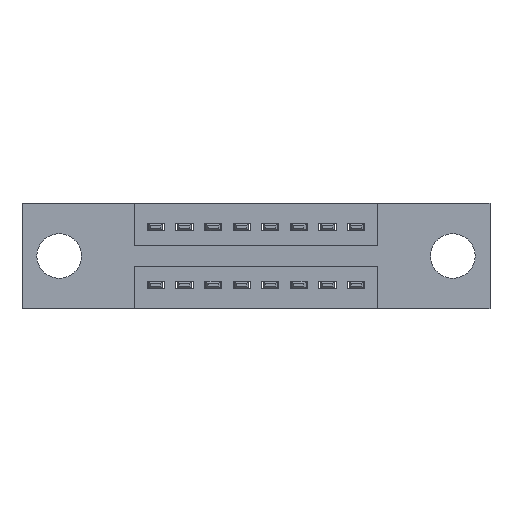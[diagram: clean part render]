
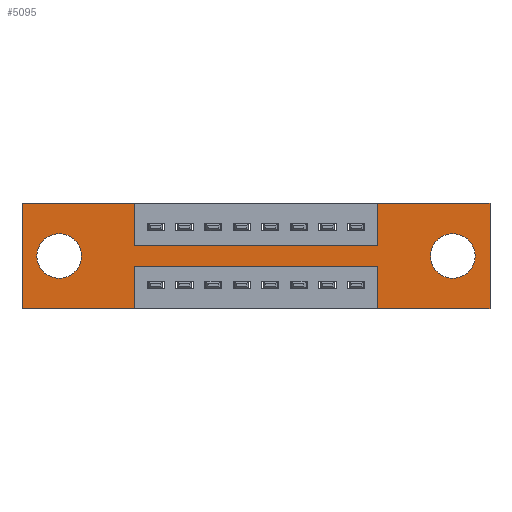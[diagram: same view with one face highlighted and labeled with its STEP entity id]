
A CAD part, front view. The second image highlights one B-rep face of the part: STEP entity #5095.
In plain terms, the highlighted planar face has unit normal (0, -1, 0).
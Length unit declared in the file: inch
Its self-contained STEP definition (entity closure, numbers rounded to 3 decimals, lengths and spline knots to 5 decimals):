
#2 = ORIENTED_EDGE ( 'NONE', *, *, #9729, .F. ) ;
#9 = CARTESIAN_POINT ( 'NONE',  ( 0.3925, 0., -0.22 ) ) ;
#35 = CARTESIAN_POINT ( 'NONE',  ( 0.13, 0., -0.185 ) ) ;
#520 = CARTESIAN_POINT ( 'NONE',  ( 1.505, 0., -0.185 ) ) ;
#651 = EDGE_CURVE ( 'NONE', #896, #5545, #6447, .T. ) ;
#751 = CARTESIAN_POINT ( 'NONE',  ( 1.2425, 0., 0. ) ) ;
#835 = CARTESIAN_POINT ( 'NONE',  ( 1.2425, 0., -0.22 ) ) ;
#842 = DIRECTION ( 'NONE',  ( 0., 0., -1. ) ) ;
#889 = CARTESIAN_POINT ( 'NONE',  ( 0., 0., 0. ) ) ;
#896 = VERTEX_POINT ( 'NONE', #7495 ) ;
#1002 = AXIS2_PLACEMENT_3D ( 'NONE', #2475, #5019, #10903 ) ;
#1089 = CARTESIAN_POINT ( 'NONE',  ( 0.3925, 0., -0.37 ) ) ;
#1166 = CARTESIAN_POINT ( 'NONE',  ( 1.2425, 0., 0. ) ) ;
#1207 = EDGE_CURVE ( 'NONE', #2217, #1642, #10713, .T. ) ;
#1431 = DIRECTION ( 'NONE',  ( 0., 0., -1. ) ) ;
#1595 = DIRECTION ( 'NONE',  ( 0., 0., 1. ) ) ;
#1608 = EDGE_LOOP ( 'NONE', ( #7619, #2039 ) ) ;
#1642 = VERTEX_POINT ( 'NONE', #8192 ) ;
#1664 = DIRECTION ( 'NONE',  ( 0., 1., 0. ) ) ;
#1670 = EDGE_CURVE ( 'NONE', #1694, #6747, #3921, .T. ) ;
#1694 = VERTEX_POINT ( 'NONE', #4988 ) ;
#1746 = ORIENTED_EDGE ( 'NONE', *, *, #651, .F. ) ;
#1755 = CARTESIAN_POINT ( 'NONE',  ( 1.2425, 0., -0.37 ) ) ;
#1835 = LINE ( 'NONE', #889, #1857 ) ;
#1857 = VECTOR ( 'NONE', #5281, 39.37008 ) ;
#1865 = CARTESIAN_POINT ( 'NONE',  ( 0.13, 0., -0.263 ) ) ;
#1866 = DIRECTION ( 'NONE',  ( 0., 0., 1. ) ) ;
#1896 = CIRCLE ( 'NONE', #1002, 0.078 ) ;
#1899 = CARTESIAN_POINT ( 'NONE',  ( 0., 0., 0. ) ) ;
#1921 = AXIS2_PLACEMENT_3D ( 'NONE', #4063, #1664, #842 ) ;
#2012 = VERTEX_POINT ( 'NONE', #1865 ) ;
#2033 = AXIS2_PLACEMENT_3D ( 'NONE', #35, #10211, #1595 ) ;
#2039 = ORIENTED_EDGE ( 'NONE', *, *, #8931, .T. ) ;
#2056 = CARTESIAN_POINT ( 'NONE',  ( 0., 0., -0.37 ) ) ;
#2217 = VERTEX_POINT ( 'NONE', #7595 ) ;
#2279 = EDGE_CURVE ( 'NONE', #5325, #8415, #7376, .T. ) ;
#2475 = CARTESIAN_POINT ( 'NONE',  ( 0.13, 0., -0.185 ) ) ;
#2544 = VERTEX_POINT ( 'NONE', #4604 ) ;
#2606 = LINE ( 'NONE', #1755, #6341 ) ;
#2649 = DIRECTION ( 'NONE',  ( -1., 0., 0. ) ) ;
#2775 = EDGE_CURVE ( 'NONE', #7670, #2217, #1835, .T. ) ;
#2829 = EDGE_CURVE ( 'NONE', #2012, #2869, #4547, .T. ) ;
#2844 = EDGE_CURVE ( 'NONE', #3544, #1694, #5229, .T. ) ;
#2869 = VERTEX_POINT ( 'NONE', #4593 ) ;
#2943 = DIRECTION ( 'NONE',  ( 0., 0., -1. ) ) ;
#3183 = EDGE_CURVE ( 'NONE', #6747, #5325, #2606, .T. ) ;
#3205 = CARTESIAN_POINT ( 'NONE',  ( 0., 0., 0. ) ) ;
#3261 = CARTESIAN_POINT ( 'NONE',  ( 0., 0., 0. ) ) ;
#3350 = EDGE_CURVE ( 'NONE', #10619, #7670, #6634, .T. ) ;
#3361 = CARTESIAN_POINT ( 'NONE',  ( 1.505, 0., -0.107 ) ) ;
#3544 = VERTEX_POINT ( 'NONE', #4455 ) ;
#3551 = EDGE_CURVE ( 'NONE', #10282, #10619, #3647, .T. ) ;
#3647 = LINE ( 'NONE', #7092, #6020 ) ;
#3796 = ORIENTED_EDGE ( 'NONE', *, *, #2775, .F. ) ;
#3841 = VERTEX_POINT ( 'NONE', #3361 ) ;
#3921 = LINE ( 'NONE', #2056, #7057 ) ;
#3968 = DIRECTION ( 'NONE',  ( 0., 1., 0. ) ) ;
#3991 = FACE_BOUND ( 'NONE', #1608, .T. ) ;
#4063 = CARTESIAN_POINT ( 'NONE',  ( 1.505, 0., -0.185 ) ) ;
#4123 = DIRECTION ( 'NONE',  ( 0., 0., 1. ) ) ;
#4149 = ORIENTED_EDGE ( 'NONE', *, *, #2829, .T. ) ;
#4242 = CIRCLE ( 'NONE', #9952, 0.078 ) ;
#4385 = DIRECTION ( 'NONE',  ( 0., 0., -1. ) ) ;
#4455 = CARTESIAN_POINT ( 'NONE',  ( 1.635, 0., 0. ) ) ;
#4547 = CIRCLE ( 'NONE', #2033, 0.078 ) ;
#4593 = CARTESIAN_POINT ( 'NONE',  ( 0.13, 0., -0.107 ) ) ;
#4604 = CARTESIAN_POINT ( 'NONE',  ( 1.505, 0., -0.263 ) ) ;
#4611 = DIRECTION ( 'NONE',  ( 0., 0., 1. ) ) ;
#4673 = VECTOR ( 'NONE', #4611, 39.37008 ) ;
#4799 = ORIENTED_EDGE ( 'NONE', *, *, #7149, .T. ) ;
#4833 = CARTESIAN_POINT ( 'NONE',  ( 0.3925, 0., 0. ) ) ;
#4952 = ORIENTED_EDGE ( 'NONE', *, *, #3350, .F. ) ;
#4988 = CARTESIAN_POINT ( 'NONE',  ( 1.635, 0., -0.37 ) ) ;
#5019 = DIRECTION ( 'NONE',  ( 0., 1., 0. ) ) ;
#5059 = DIRECTION ( 'NONE',  ( 1., 0., 0. ) ) ;
#5095 = ADVANCED_FACE ( 'NONE', ( #3991, #7643, #6739 ), #5897, .T. ) ;
#5179 = VECTOR ( 'NONE', #5905, 39.37008 ) ;
#5229 = LINE ( 'NONE', #8652, #7979 ) ;
#5281 = DIRECTION ( 'NONE',  ( 1., 0., 0. ) ) ;
#5325 = VERTEX_POINT ( 'NONE', #835 ) ;
#5482 = ORIENTED_EDGE ( 'NONE', *, *, #1207, .F. ) ;
#5545 = VERTEX_POINT ( 'NONE', #751 ) ;
#5653 = AXIS2_PLACEMENT_3D ( 'NONE', #10821, #7526, #7580 ) ;
#5655 = EDGE_LOOP ( 'NONE', ( #4799, #4149 ) ) ;
#5760 = DIRECTION ( 'NONE',  ( 0., 0., -1. ) ) ;
#5807 = VECTOR ( 'NONE', #2943, 39.37008 ) ;
#5897 = PLANE ( 'NONE',  #5653 ) ;
#5905 = DIRECTION ( 'NONE',  ( 1., 0., 0. ) ) ;
#6020 = VECTOR ( 'NONE', #2649, 39.37008 ) ;
#6064 = ORIENTED_EDGE ( 'NONE', *, *, #7579, .F. ) ;
#6135 = ORIENTED_EDGE ( 'NONE', *, *, #2844, .F. ) ;
#6341 = VECTOR ( 'NONE', #1866, 39.37008 ) ;
#6447 = LINE ( 'NONE', #1166, #4673 ) ;
#6548 = DIRECTION ( 'NONE',  ( -1., 0., 0. ) ) ;
#6554 = EDGE_CURVE ( 'NONE', #3841, #2544, #4242, .T. ) ;
#6578 = DIRECTION ( 'NONE',  ( -1., 0., 0. ) ) ;
#6634 = LINE ( 'NONE', #3261, #9245 ) ;
#6674 = ORIENTED_EDGE ( 'NONE', *, *, #3551, .F. ) ;
#6739 = FACE_OUTER_BOUND ( 'NONE', #8005, .T. ) ;
#6747 = VERTEX_POINT ( 'NONE', #8576 ) ;
#6752 = LINE ( 'NONE', #3205, #5179 ) ;
#7057 = VECTOR ( 'NONE', #6548, 39.37008 ) ;
#7092 = CARTESIAN_POINT ( 'NONE',  ( 0., 0., -0.37 ) ) ;
#7149 = EDGE_CURVE ( 'NONE', #2869, #2012, #1896, .T. ) ;
#7178 = CARTESIAN_POINT ( 'NONE',  ( 0.3925, 0., -0.37 ) ) ;
#7334 = ORIENTED_EDGE ( 'NONE', *, *, #3183, .F. ) ;
#7376 = LINE ( 'NONE', #10835, #9213 ) ;
#7495 = CARTESIAN_POINT ( 'NONE',  ( 1.2425, 0., -0.15 ) ) ;
#7526 = DIRECTION ( 'NONE',  ( 0., -1., 0. ) ) ;
#7579 = EDGE_CURVE ( 'NONE', #1642, #896, #8375, .T. ) ;
#7580 = DIRECTION ( 'NONE',  ( 0., 0., -1. ) ) ;
#7595 = CARTESIAN_POINT ( 'NONE',  ( 0.3925, 0., 0. ) ) ;
#7619 = ORIENTED_EDGE ( 'NONE', *, *, #6554, .T. ) ;
#7643 = FACE_BOUND ( 'NONE', #5655, .T. ) ;
#7670 = VERTEX_POINT ( 'NONE', #1899 ) ;
#7692 = CIRCLE ( 'NONE', #1921, 0.078 ) ;
#7883 = ORIENTED_EDGE ( 'NONE', *, *, #8904, .F. ) ;
#7895 = CARTESIAN_POINT ( 'NONE',  ( 0., 0., -0.37 ) ) ;
#7979 = VECTOR ( 'NONE', #4385, 39.37008 ) ;
#8005 = EDGE_LOOP ( 'NONE', ( #2, #10016, #7334, #9868, #6135, #7883, #1746, #6064, #5482, #3796, #4952, #6674 ) ) ;
#8123 = LINE ( 'NONE', #1089, #5807 ) ;
#8192 = CARTESIAN_POINT ( 'NONE',  ( 0.3925, 0., -0.15 ) ) ;
#8375 = LINE ( 'NONE', #10164, #9634 ) ;
#8415 = VERTEX_POINT ( 'NONE', #9 ) ;
#8576 = CARTESIAN_POINT ( 'NONE',  ( 1.2425, 0., -0.37 ) ) ;
#8652 = CARTESIAN_POINT ( 'NONE',  ( 1.635, 0., 0. ) ) ;
#8904 = EDGE_CURVE ( 'NONE', #5545, #3544, #6752, .T. ) ;
#8931 = EDGE_CURVE ( 'NONE', #2544, #3841, #7692, .T. ) ;
#9213 = VECTOR ( 'NONE', #6578, 39.37008 ) ;
#9245 = VECTOR ( 'NONE', #4123, 39.37008 ) ;
#9550 = VECTOR ( 'NONE', #1431, 39.37008 ) ;
#9634 = VECTOR ( 'NONE', #5059, 39.37008 ) ;
#9729 = EDGE_CURVE ( 'NONE', #8415, #10282, #8123, .T. ) ;
#9868 = ORIENTED_EDGE ( 'NONE', *, *, #1670, .F. ) ;
#9952 = AXIS2_PLACEMENT_3D ( 'NONE', #520, #3968, #5760 ) ;
#10016 = ORIENTED_EDGE ( 'NONE', *, *, #2279, .F. ) ;
#10164 = CARTESIAN_POINT ( 'NONE',  ( 0.3925, 0., -0.15 ) ) ;
#10211 = DIRECTION ( 'NONE',  ( 0., 1., 0. ) ) ;
#10282 = VERTEX_POINT ( 'NONE', #7178 ) ;
#10619 = VERTEX_POINT ( 'NONE', #7895 ) ;
#10713 = LINE ( 'NONE', #4833, #9550 ) ;
#10821 = CARTESIAN_POINT ( 'NONE',  ( 0., 0., -0.37 ) ) ;
#10835 = CARTESIAN_POINT ( 'NONE',  ( 0.3925, 0., -0.22 ) ) ;
#10903 = DIRECTION ( 'NONE',  ( 0., 0., 1. ) ) ;
